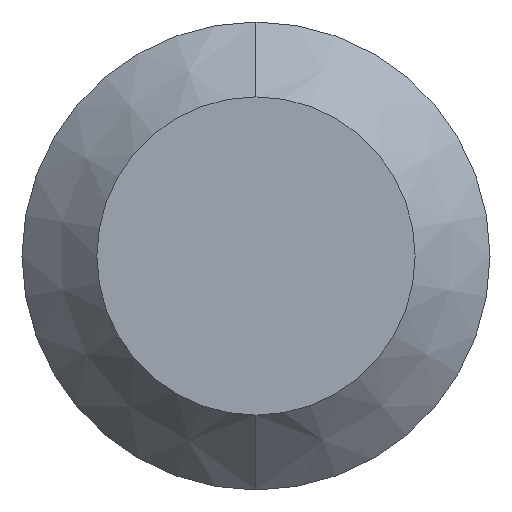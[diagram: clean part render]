
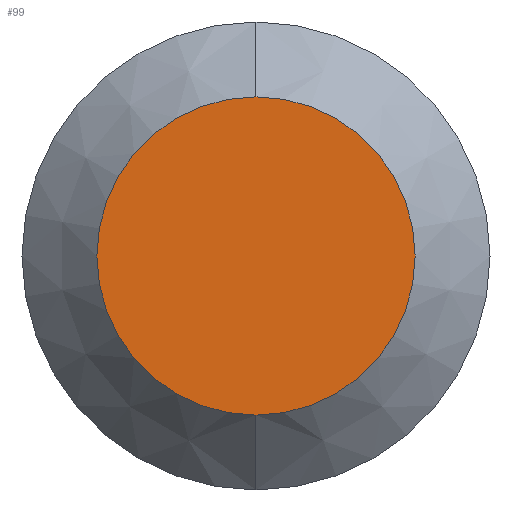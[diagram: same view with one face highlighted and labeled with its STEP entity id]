
A CAD part, left-side view. The second image highlights one B-rep face of the part: STEP entity #99.
In plain terms, the highlighted planar face has unit normal (-1, 0, 0).
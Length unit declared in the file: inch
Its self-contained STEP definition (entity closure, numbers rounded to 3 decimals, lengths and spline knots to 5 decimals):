
#3 = DIRECTION ( 'NONE',  ( 1., 0., 0. ) ) ;
#14 = ORIENTED_EDGE ( 'NONE', *, *, #240, .T. ) ;
#17 = FACE_OUTER_BOUND ( 'NONE', #185, .T. ) ;
#20 = DIRECTION ( 'NONE',  ( 0., 0., -1. ) ) ;
#26 = DIRECTION ( 'NONE',  ( 0., 0., -1. ) ) ;
#40 = CARTESIAN_POINT ( 'NONE',  ( 0., 0., 0. ) ) ;
#50 = AXIS2_PLACEMENT_3D ( 'NONE', #201, #3, #20 ) ;
#56 = DIRECTION ( 'NONE',  ( -1., 0., 0. ) ) ;
#83 = CARTESIAN_POINT ( 'NONE',  ( 0., 0., 0. ) ) ;
#95 = PLANE ( 'NONE',  #50 ) ;
#99 = ADVANCED_FACE ( 'NONE', ( #17 ), #95, .F. ) ;
#100 = ORIENTED_EDGE ( 'NONE', *, *, #107, .T. ) ;
#107 = EDGE_CURVE ( 'NONE', #208, #124, #242, .T. ) ;
#114 = DIRECTION ( 'NONE',  ( 0., 0., -1. ) ) ;
#124 = VERTEX_POINT ( 'NONE', #211 ) ;
#136 = AXIS2_PLACEMENT_3D ( 'NONE', #40, #216, #114 ) ;
#174 = AXIS2_PLACEMENT_3D ( 'NONE', #83, #56, #26 ) ;
#185 = EDGE_LOOP ( 'NONE', ( #100, #14 ) ) ;
#196 = CARTESIAN_POINT ( 'NONE',  ( 0., 0., -0.0425 ) ) ;
#201 = CARTESIAN_POINT ( 'NONE',  ( 0., 0., 0. ) ) ;
#208 = VERTEX_POINT ( 'NONE', #196 ) ;
#209 = CIRCLE ( 'NONE', #174, 0.0425 ) ;
#211 = CARTESIAN_POINT ( 'NONE',  ( 0., 0., 0.0425 ) ) ;
#216 = DIRECTION ( 'NONE',  ( -1., 0., 0. ) ) ;
#240 = EDGE_CURVE ( 'NONE', #124, #208, #209, .T. ) ;
#242 = CIRCLE ( 'NONE', #136, 0.0425 ) ;
